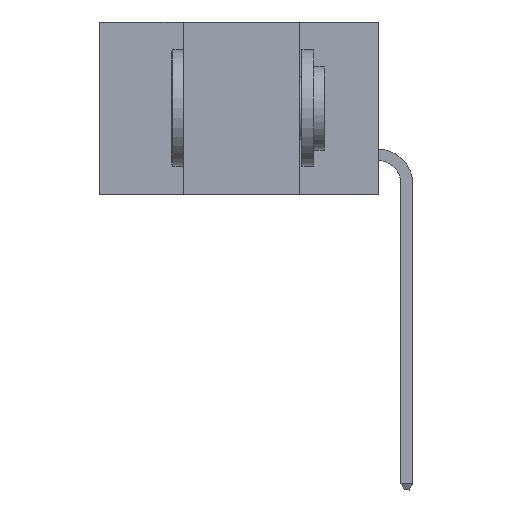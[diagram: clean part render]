
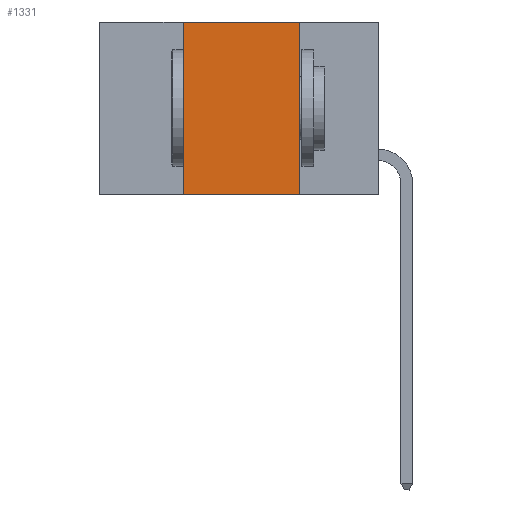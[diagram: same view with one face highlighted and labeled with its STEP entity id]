
A CAD part, left-side view. The second image highlights one B-rep face of the part: STEP entity #1331.
In plain terms, the highlighted planar face has unit normal (-1, 0, 0).
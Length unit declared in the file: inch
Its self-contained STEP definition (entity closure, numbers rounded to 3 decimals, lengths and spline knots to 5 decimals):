
#451 = EDGE_CURVE ( 'NONE', #12210, #17119, #9365, .T. ) ;
#827 = VECTOR ( 'NONE', #7671, 39.37008 ) ;
#1331 = ADVANCED_FACE ( 'NONE', ( #9605 ), #9029, .F. ) ;
#1368 = VERTEX_POINT ( 'NONE', #15794 ) ;
#1688 = DIRECTION ( 'NONE',  ( 0., 0., -1. ) ) ;
#1711 = DIRECTION ( 'NONE',  ( 1., 0., 0. ) ) ;
#1950 = VECTOR ( 'NONE', #16447, 39.37008 ) ;
#3364 = CARTESIAN_POINT ( 'NONE',  ( 0., 0.6, -0.37 ) ) ;
#4720 = ORIENTED_EDGE ( 'NONE', *, *, #9835, .F. ) ;
#4988 = ORIENTED_EDGE ( 'NONE', *, *, #7668, .T. ) ;
#6703 = CARTESIAN_POINT ( 'NONE',  ( 0., 0.17, 0. ) ) ;
#7668 = EDGE_CURVE ( 'NONE', #1368, #17119, #11975, .T. ) ;
#7671 = DIRECTION ( 'NONE',  ( 0., -1., 0. ) ) ;
#7755 = AXIS2_PLACEMENT_3D ( 'NONE', #16566, #1711, #1688 ) ;
#7801 = CARTESIAN_POINT ( 'NONE',  ( 0., 0.17, -0.37 ) ) ;
#8310 = VECTOR ( 'NONE', #9253, 39.37008 ) ;
#8713 = LINE ( 'NONE', #14739, #8310 ) ;
#8889 = EDGE_CURVE ( 'NONE', #16080, #12210, #8713, .T. ) ;
#9029 = PLANE ( 'NONE',  #7755 ) ;
#9253 = DIRECTION ( 'NONE',  ( 0., -1., 0. ) ) ;
#9365 = LINE ( 'NONE', #16296, #1950 ) ;
#9523 = VECTOR ( 'NONE', #13106, 39.37008 ) ;
#9605 = FACE_OUTER_BOUND ( 'NONE', #10091, .T. ) ;
#9835 = EDGE_CURVE ( 'NONE', #1368, #16080, #13210, .T. ) ;
#10091 = EDGE_LOOP ( 'NONE', ( #13564, #16783, #4720, #4988 ) ) ;
#11735 = CARTESIAN_POINT ( 'NONE',  ( 0., 0.42, 0. ) ) ;
#11975 = LINE ( 'NONE', #3364, #827 ) ;
#12210 = VERTEX_POINT ( 'NONE', #6703 ) ;
#13106 = DIRECTION ( 'NONE',  ( 0., 0., 1. ) ) ;
#13210 = LINE ( 'NONE', #11735, #9523 ) ;
#13564 = ORIENTED_EDGE ( 'NONE', *, *, #451, .F. ) ;
#14739 = CARTESIAN_POINT ( 'NONE',  ( 0., 0.6, 0. ) ) ;
#15794 = CARTESIAN_POINT ( 'NONE',  ( 0., 0.42, -0.37 ) ) ;
#16080 = VERTEX_POINT ( 'NONE', #17962 ) ;
#16296 = CARTESIAN_POINT ( 'NONE',  ( 0., 0.17, 0. ) ) ;
#16447 = DIRECTION ( 'NONE',  ( 0., 0., -1. ) ) ;
#16566 = CARTESIAN_POINT ( 'NONE',  ( 0., 0.6, 0. ) ) ;
#16783 = ORIENTED_EDGE ( 'NONE', *, *, #8889, .F. ) ;
#17119 = VERTEX_POINT ( 'NONE', #7801 ) ;
#17962 = CARTESIAN_POINT ( 'NONE',  ( 0., 0.42, 0. ) ) ;
